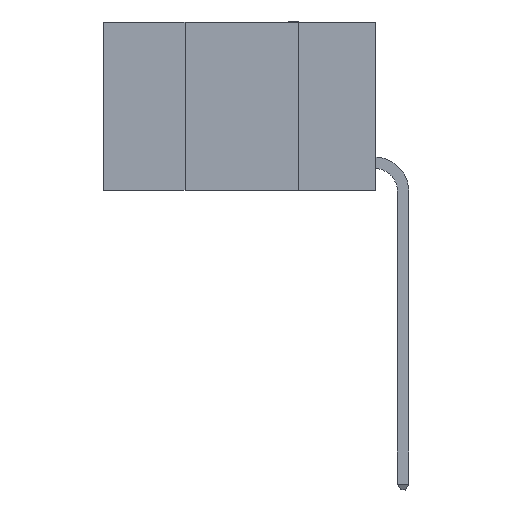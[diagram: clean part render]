
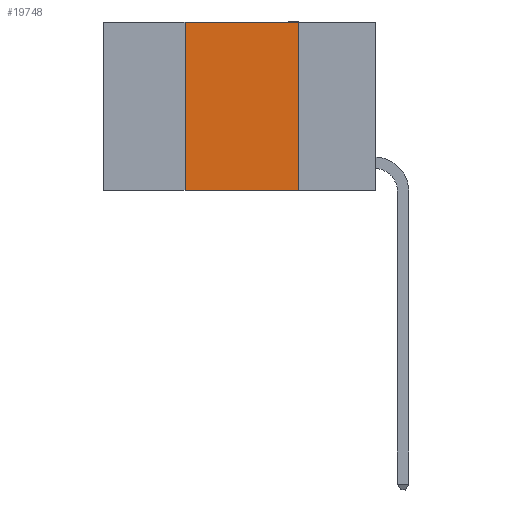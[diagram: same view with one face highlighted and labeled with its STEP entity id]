
A CAD part, left-side view. The second image highlights one B-rep face of the part: STEP entity #19748.
In plain terms, the highlighted planar face has unit normal (-1, 0, 0).
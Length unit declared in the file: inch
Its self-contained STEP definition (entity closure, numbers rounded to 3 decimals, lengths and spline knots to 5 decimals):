
#2329 = DIRECTION ( 'NONE',  ( 0., 0., -1. ) ) ;
#3480 = LINE ( 'NONE', #17321, #17918 ) ;
#5088 = CARTESIAN_POINT ( 'NONE',  ( 0., 0.6, -0.37 ) ) ;
#5338 = LINE ( 'NONE', #5088, #14777 ) ;
#5439 = CARTESIAN_POINT ( 'NONE',  ( 0., 0.42, 0. ) ) ;
#5510 = LINE ( 'NONE', #19606, #10028 ) ;
#5683 = ORIENTED_EDGE ( 'NONE', *, *, #18630, .F. ) ;
#5720 = PLANE ( 'NONE',  #15732 ) ;
#6292 = CARTESIAN_POINT ( 'NONE',  ( 0., 0.17, -0.37 ) ) ;
#7405 = DIRECTION ( 'NONE',  ( 0., 0., -1. ) ) ;
#7728 = EDGE_CURVE ( 'NONE', #10762, #17698, #5510, .T. ) ;
#7754 = LINE ( 'NONE', #10740, #11188 ) ;
#9597 = VERTEX_POINT ( 'NONE', #9705 ) ;
#9705 = CARTESIAN_POINT ( 'NONE',  ( 0., 0.42, -0.37 ) ) ;
#9775 = DIRECTION ( 'NONE',  ( 0., -1., 0. ) ) ;
#10028 = VECTOR ( 'NONE', #9775, 39.37008 ) ;
#10724 = ORIENTED_EDGE ( 'NONE', *, *, #7728, .F. ) ;
#10740 = CARTESIAN_POINT ( 'NONE',  ( 0., 0.42, 0. ) ) ;
#10762 = VERTEX_POINT ( 'NONE', #5439 ) ;
#11090 = EDGE_LOOP ( 'NONE', ( #5683, #10724, #19441, #11772 ) ) ;
#11188 = VECTOR ( 'NONE', #14053, 39.37008 ) ;
#11772 = ORIENTED_EDGE ( 'NONE', *, *, #20098, .T. ) ;
#12072 = EDGE_CURVE ( 'NONE', #9597, #10762, #7754, .T. ) ;
#12505 = DIRECTION ( 'NONE',  ( 1., 0., 0. ) ) ;
#14053 = DIRECTION ( 'NONE',  ( 0., 0., 1. ) ) ;
#14449 = VERTEX_POINT ( 'NONE', #6292 ) ;
#14777 = VECTOR ( 'NONE', #16749, 39.37008 ) ;
#15732 = AXIS2_PLACEMENT_3D ( 'NONE', #20601, #12505, #2329 ) ;
#16749 = DIRECTION ( 'NONE',  ( 0., -1., 0. ) ) ;
#17090 = FACE_OUTER_BOUND ( 'NONE', #11090, .T. ) ;
#17321 = CARTESIAN_POINT ( 'NONE',  ( 0., 0.17, 0. ) ) ;
#17698 = VERTEX_POINT ( 'NONE', #21387 ) ;
#17918 = VECTOR ( 'NONE', #7405, 39.37008 ) ;
#18630 = EDGE_CURVE ( 'NONE', #17698, #14449, #3480, .T. ) ;
#19441 = ORIENTED_EDGE ( 'NONE', *, *, #12072, .F. ) ;
#19606 = CARTESIAN_POINT ( 'NONE',  ( 0., 0.6, 0. ) ) ;
#19748 = ADVANCED_FACE ( 'NONE', ( #17090 ), #5720, .F. ) ;
#20098 = EDGE_CURVE ( 'NONE', #9597, #14449, #5338, .T. ) ;
#20601 = CARTESIAN_POINT ( 'NONE',  ( 0., 0.6, 0. ) ) ;
#21387 = CARTESIAN_POINT ( 'NONE',  ( 0., 0.17, 0. ) ) ;
